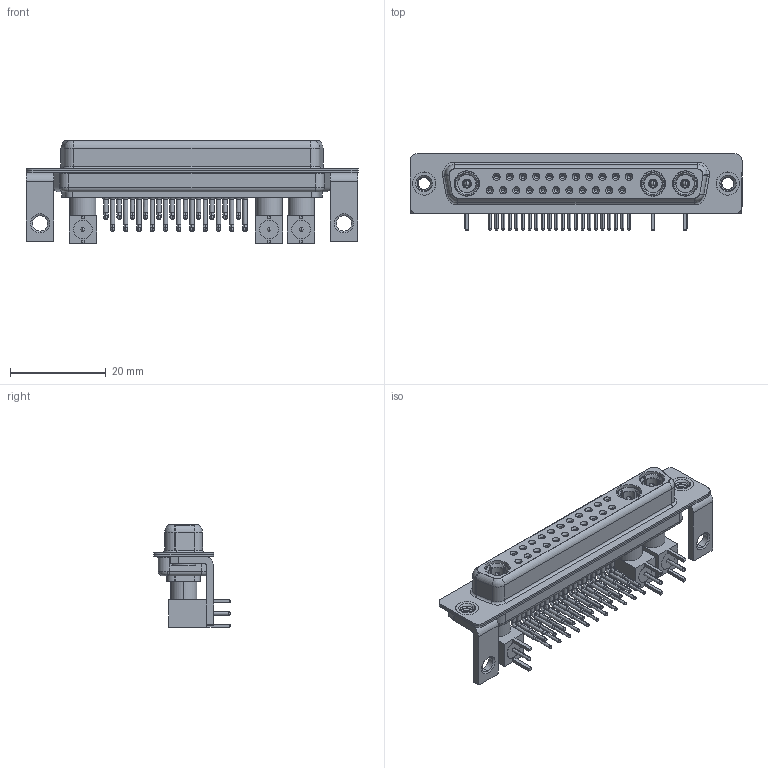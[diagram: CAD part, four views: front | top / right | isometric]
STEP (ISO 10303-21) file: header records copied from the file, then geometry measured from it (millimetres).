
FILE_DESCRIPTION (( 'STEP AP203' ), '1' );
FILE_NAME ('630-25W3240-5NC.STEP', '2022-06-07T03:43:48', ( '' ), ( '' ), 'SwSTEP 2.0', 'SolidWorks 2020', '' );
FILE_SCHEMA (( 'CONFIG_CONTROL_DESIGN' ));
Length unit declared in the file: millimetre
Products named in the file (17): 630Combo Threaded Rivet_B; 630Combo Contact Row 2; Pin_RA; Insulator Pin_Straight PC Tail; 630-25W3240-5NC; Insulator RA Pin; Co-Ax Plug_RA PC Tail; 630Combo Stabilizer Bracket; RA Back Shell; 630Combo Housing_25W3; Co-Ax Plug Assy_RA; 630Combo Shell Front_37 Contacts; Locking Collar; 630Combo Contact Row 1; 630Combo Shell Rear_37 Contacts
Assembly tree (50 placements, depth 3):
  630-25W3240-5NC
    630Combo Housing_25W3
    630Combo Shell Front_37 Contacts
    630Combo Shell Rear_37 Contacts
    630Combo Threaded Rivet_B  x2
    630Combo Stabilizer Bracket  x2
    Co-Ax Plug Assy_RA
      Co-Ax Plug_RA PC Tail
      Insulator Pin_Straight PC Tail
      Pin_RA
      Locking Collar
      RA Back Shell
      Insulator RA Pin
    Co-Ax Plug Assy_RA
      Co-Ax Plug_RA PC Tail
      Insulator Pin_Straight PC Tail
      Pin_RA
      Locking Collar
      RA Back Shell
      Insulator RA Pin
    Co-Ax Plug Assy_RA
      Co-Ax Plug_RA PC Tail
      Insulator Pin_Straight PC Tail
      Pin_RA
      Locking Collar
      RA Back Shell
      Insulator RA Pin
    630Combo Contact Row 1  x11
    630Combo Contact Row 2  x11
Bounding box: 69.4 x 16 x 21.41 mm (x, y, z)
Volume: 6434.9 mm3; surface area: 15168 mm2
Topology: 47 solids, 47 shells, 1987 faces, 4958 edges, 3116 vertices
Faces by surface type: cylinder 856, plane 618, cone 329, bspline 97, torus 75, sphere 12
Entity records: 28159 total; most frequent: CARTESIAN_POINT 5968, DIRECTION 4483, ORIENTED_EDGE 3778, EDGE_CURVE 1889, AXIS2_PLACEMENT_3D 1852, VERTEX_POINT 1203, CIRCLE 999, EDGE_LOOP 982
